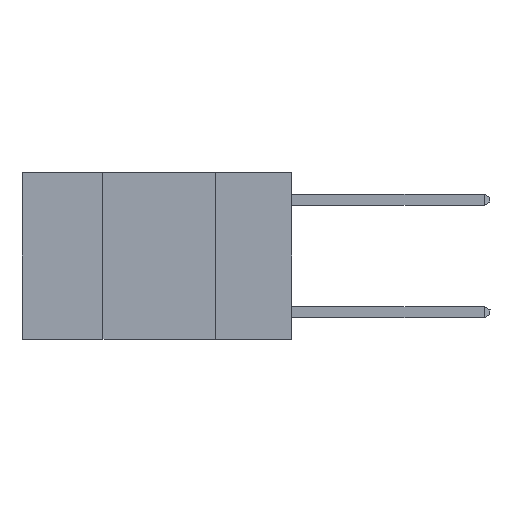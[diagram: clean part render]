
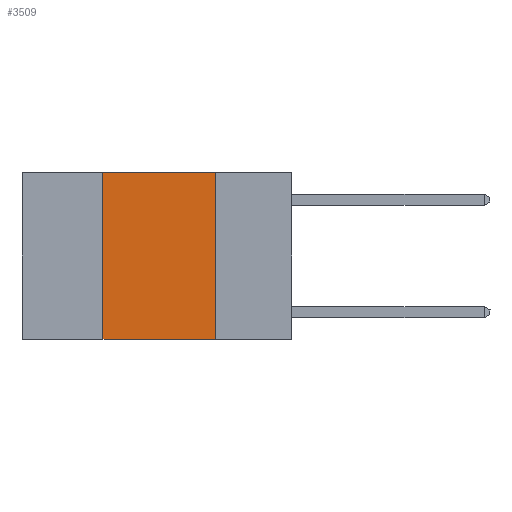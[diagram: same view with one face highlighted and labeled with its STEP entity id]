
A CAD part, left-side view. The second image highlights one B-rep face of the part: STEP entity #3509.
In plain terms, the highlighted planar face has unit normal (-1, 0, 0).
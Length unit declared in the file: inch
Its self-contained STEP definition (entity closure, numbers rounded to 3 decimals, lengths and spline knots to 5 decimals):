
#487 = DIRECTION ( 'NONE',  ( 0., 0., -1. ) ) ;
#491 = DIRECTION ( 'NONE',  ( 1., 0., 0. ) ) ;
#518 = PLANE ( 'NONE',  #6180 ) ;
#578 = CARTESIAN_POINT ( 'NONE',  ( 0., 0.6, 0. ) ) ;
#779 = CARTESIAN_POINT ( 'NONE',  ( 0., 0.17, 0. ) ) ;
#784 = ORIENTED_EDGE ( 'NONE', *, *, #8621, .F. ) ;
#1179 = LINE ( 'NONE', #7599, #5125 ) ;
#1361 = CARTESIAN_POINT ( 'NONE',  ( 0., 0.42, 0. ) ) ;
#1439 = VECTOR ( 'NONE', #6825, 39.37008 ) ;
#1772 = CARTESIAN_POINT ( 'NONE',  ( 0., 0.42, -0.37 ) ) ;
#1799 = ORIENTED_EDGE ( 'NONE', *, *, #5333, .T. ) ;
#1978 = LINE ( 'NONE', #6486, #6199 ) ;
#2549 = DIRECTION ( 'NONE',  ( 0., -1., 0. ) ) ;
#2641 = ORIENTED_EDGE ( 'NONE', *, *, #7454, .F. ) ;
#2998 = VECTOR ( 'NONE', #3159, 39.37008 ) ;
#3159 = DIRECTION ( 'NONE',  ( 0., -1., 0. ) ) ;
#3509 = ADVANCED_FACE ( 'NONE', ( #6502 ), #518, .F. ) ;
#3518 = LINE ( 'NONE', #5353, #1439 ) ;
#4153 = EDGE_LOOP ( 'NONE', ( #4623, #784, #2641, #1799 ) ) ;
#4260 = CARTESIAN_POINT ( 'NONE',  ( 0., 0.17, -0.37 ) ) ;
#4623 = ORIENTED_EDGE ( 'NONE', *, *, #9754, .F. ) ;
#5125 = VECTOR ( 'NONE', #8340, 39.37008 ) ;
#5180 = LINE ( 'NONE', #5574, #2998 ) ;
#5236 = VERTEX_POINT ( 'NONE', #779 ) ;
#5333 = EDGE_CURVE ( 'NONE', #7061, #8623, #5180, .T. ) ;
#5353 = CARTESIAN_POINT ( 'NONE',  ( 0., 0.42, 0. ) ) ;
#5574 = CARTESIAN_POINT ( 'NONE',  ( 0., 0.6, -0.37 ) ) ;
#6180 = AXIS2_PLACEMENT_3D ( 'NONE', #578, #491, #487 ) ;
#6199 = VECTOR ( 'NONE', #2549, 39.37008 ) ;
#6486 = CARTESIAN_POINT ( 'NONE',  ( 0., 0.6, 0. ) ) ;
#6502 = FACE_OUTER_BOUND ( 'NONE', #4153, .T. ) ;
#6825 = DIRECTION ( 'NONE',  ( 0., 0., 1. ) ) ;
#7061 = VERTEX_POINT ( 'NONE', #1772 ) ;
#7454 = EDGE_CURVE ( 'NONE', #7061, #9645, #3518, .T. ) ;
#7599 = CARTESIAN_POINT ( 'NONE',  ( 0., 0.17, 0. ) ) ;
#8340 = DIRECTION ( 'NONE',  ( 0., 0., -1. ) ) ;
#8621 = EDGE_CURVE ( 'NONE', #9645, #5236, #1978, .T. ) ;
#8623 = VERTEX_POINT ( 'NONE', #4260 ) ;
#9645 = VERTEX_POINT ( 'NONE', #1361 ) ;
#9754 = EDGE_CURVE ( 'NONE', #5236, #8623, #1179, .T. ) ;
